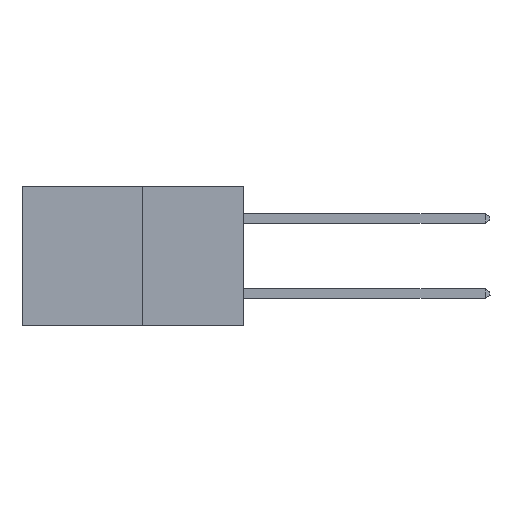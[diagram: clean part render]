
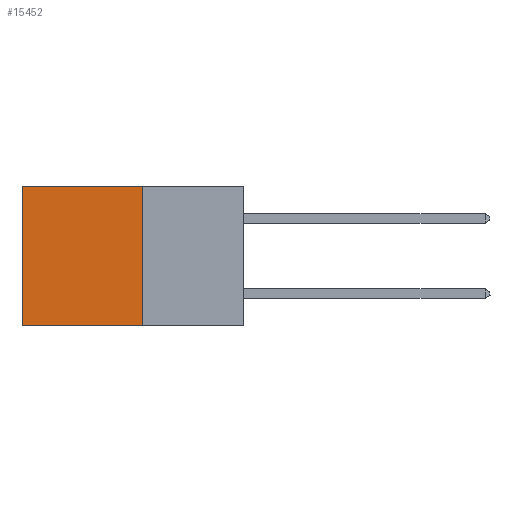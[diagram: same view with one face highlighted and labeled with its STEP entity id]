
A CAD part, left-side view. The second image highlights one B-rep face of the part: STEP entity #15452.
In plain terms, the highlighted planar face has unit normal (-1, 0, 0).
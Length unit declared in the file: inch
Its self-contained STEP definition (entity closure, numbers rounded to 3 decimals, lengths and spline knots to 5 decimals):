
#612 = DIRECTION ( 'NONE',  ( 1., 0., 0. ) ) ;
#703 = VECTOR ( 'NONE', #11799, 39.37008 ) ;
#1111 = LINE ( 'NONE', #4303, #703 ) ;
#1213 = EDGE_LOOP ( 'NONE', ( #14912, #13693, #5201, #1510 ) ) ;
#1454 = AXIS2_PLACEMENT_3D ( 'NONE', #8203, #612, #9460 ) ;
#1510 = ORIENTED_EDGE ( 'NONE', *, *, #7900, .T. ) ;
#2375 = VERTEX_POINT ( 'NONE', #12218 ) ;
#2690 = LINE ( 'NONE', #8913, #15621 ) ;
#2761 = CARTESIAN_POINT ( 'NONE',  ( 0.277, 0.27, -0.37 ) ) ;
#3313 = FACE_OUTER_BOUND ( 'NONE', #1213, .T. ) ;
#3335 = DIRECTION ( 'NONE',  ( 0., 0., -1. ) ) ;
#3430 = EDGE_CURVE ( 'NONE', #8632, #4120, #7495, .T. ) ;
#4120 = VERTEX_POINT ( 'NONE', #2761 ) ;
#4303 = CARTESIAN_POINT ( 'NONE',  ( 0.277, 0.27, -0.37 ) ) ;
#5201 = ORIENTED_EDGE ( 'NONE', *, *, #3430, .F. ) ;
#7265 = CARTESIAN_POINT ( 'NONE',  ( 0.277, 0.59, 0. ) ) ;
#7495 = LINE ( 'NONE', #12305, #13746 ) ;
#7900 = EDGE_CURVE ( 'NONE', #8632, #13154, #2690, .T. ) ;
#8203 = CARTESIAN_POINT ( 'NONE',  ( 0.277, 0.27, -0.37 ) ) ;
#8610 = DIRECTION ( 'NONE',  ( 0., 0., -1. ) ) ;
#8632 = VERTEX_POINT ( 'NONE', #9107 ) ;
#8913 = CARTESIAN_POINT ( 'NONE',  ( 0.277, 0.27, 0. ) ) ;
#9107 = CARTESIAN_POINT ( 'NONE',  ( 0.277, 0.27, 0. ) ) ;
#9460 = DIRECTION ( 'NONE',  ( 0., 0., -1. ) ) ;
#10201 = VECTOR ( 'NONE', #3335, 39.37008 ) ;
#11799 = DIRECTION ( 'NONE',  ( 0., 1., 0. ) ) ;
#12218 = CARTESIAN_POINT ( 'NONE',  ( 0.277, 0.59, -0.37 ) ) ;
#12305 = CARTESIAN_POINT ( 'NONE',  ( 0.277, 0.27, -0.37 ) ) ;
#12666 = DIRECTION ( 'NONE',  ( 0., 1., 0. ) ) ;
#13154 = VERTEX_POINT ( 'NONE', #7265 ) ;
#13526 = LINE ( 'NONE', #14562, #10201 ) ;
#13693 = ORIENTED_EDGE ( 'NONE', *, *, #15414, .F. ) ;
#13746 = VECTOR ( 'NONE', #8610, 39.37008 ) ;
#14562 = CARTESIAN_POINT ( 'NONE',  ( 0.277, 0.59, -0.37 ) ) ;
#14751 = EDGE_CURVE ( 'NONE', #13154, #2375, #13526, .T. ) ;
#14912 = ORIENTED_EDGE ( 'NONE', *, *, #14751, .T. ) ;
#15414 = EDGE_CURVE ( 'NONE', #4120, #2375, #1111, .T. ) ;
#15452 = ADVANCED_FACE ( 'NONE', ( #3313 ), #15673, .F. ) ;
#15621 = VECTOR ( 'NONE', #12666, 39.37008 ) ;
#15673 = PLANE ( 'NONE',  #1454 ) ;
